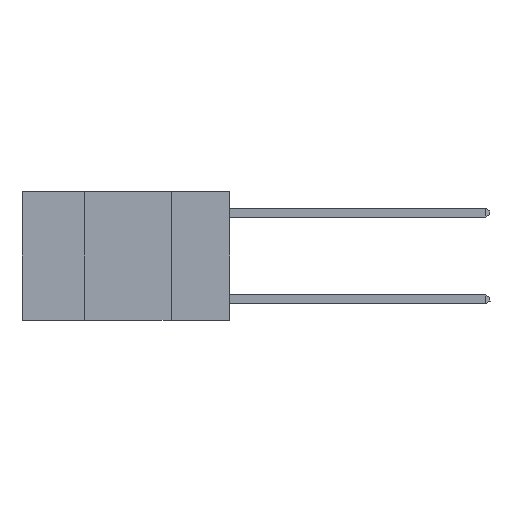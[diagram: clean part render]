
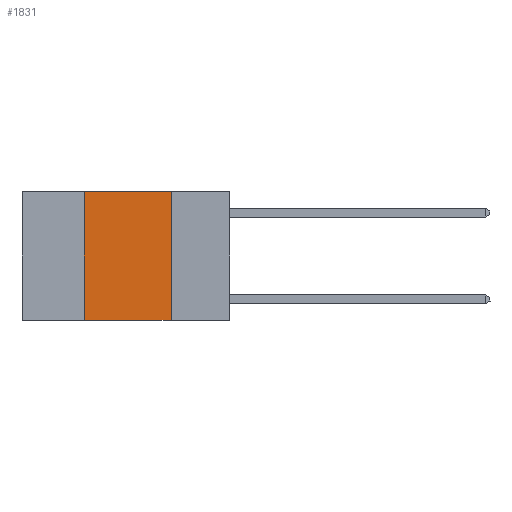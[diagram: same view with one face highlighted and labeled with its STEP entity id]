
A CAD part, left-side view. The second image highlights one B-rep face of the part: STEP entity #1831.
In plain terms, the highlighted planar face has unit normal (-1, 0, 0).
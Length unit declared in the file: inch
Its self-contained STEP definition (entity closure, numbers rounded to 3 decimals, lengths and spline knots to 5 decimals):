
#121 = DIRECTION ( 'NONE',  ( 0., -1., 0. ) ) ;
#196 = ORIENTED_EDGE ( 'NONE', *, *, #12765, .F. ) ;
#263 = ORIENTED_EDGE ( 'NONE', *, *, #1273, .F. ) ;
#486 = EDGE_CURVE ( 'NONE', #14666, #20939, #19412, .T. ) ;
#539 = ORIENTED_EDGE ( 'NONE', *, *, #14400, .F. ) ;
#696 = ORIENTED_EDGE ( 'NONE', *, *, #486, .T. ) ;
#1133 = CARTESIAN_POINT ( 'NONE',  ( 0., 0.42, 0. ) ) ;
#1273 = EDGE_CURVE ( 'NONE', #9100, #5778, #14840, .T. ) ;
#1831 = ADVANCED_FACE ( 'NONE', ( #8430 ), #6531, .F. ) ;
#2457 = CARTESIAN_POINT ( 'NONE',  ( 0., 0.17, 0. ) ) ;
#3127 = CARTESIAN_POINT ( 'NONE',  ( 0., 0.6, 0. ) ) ;
#5778 = VERTEX_POINT ( 'NONE', #11960 ) ;
#6531 = PLANE ( 'NONE',  #10584 ) ;
#8238 = DIRECTION ( 'NONE',  ( 1., 0., 0. ) ) ;
#8430 = FACE_OUTER_BOUND ( 'NONE', #15320, .T. ) ;
#9100 = VERTEX_POINT ( 'NONE', #18956 ) ;
#9338 = LINE ( 'NONE', #2457, #16478 ) ;
#10584 = AXIS2_PLACEMENT_3D ( 'NONE', #3127, #8238, #19606 ) ;
#11960 = CARTESIAN_POINT ( 'NONE',  ( 0., 0.17, 0. ) ) ;
#12765 = EDGE_CURVE ( 'NONE', #5778, #20939, #9338, .T. ) ;
#12866 = DIRECTION ( 'NONE',  ( 0., 0., 1. ) ) ;
#13120 = VECTOR ( 'NONE', #12866, 39.37008 ) ;
#13431 = CARTESIAN_POINT ( 'NONE',  ( 0., 0.42, -0.37 ) ) ;
#14050 = DIRECTION ( 'NONE',  ( 0., -1., 0. ) ) ;
#14340 = VECTOR ( 'NONE', #121, 39.37008 ) ;
#14400 = EDGE_CURVE ( 'NONE', #14666, #9100, #17918, .T. ) ;
#14666 = VERTEX_POINT ( 'NONE', #13431 ) ;
#14840 = LINE ( 'NONE', #17316, #14340 ) ;
#15138 = VECTOR ( 'NONE', #14050, 39.37008 ) ;
#15320 = EDGE_LOOP ( 'NONE', ( #196, #263, #539, #696 ) ) ;
#15321 = CARTESIAN_POINT ( 'NONE',  ( 0., 0.6, -0.37 ) ) ;
#15734 = DIRECTION ( 'NONE',  ( 0., 0., -1. ) ) ;
#16478 = VECTOR ( 'NONE', #15734, 39.37008 ) ;
#17316 = CARTESIAN_POINT ( 'NONE',  ( 0., 0.6, 0. ) ) ;
#17918 = LINE ( 'NONE', #1133, #13120 ) ;
#18956 = CARTESIAN_POINT ( 'NONE',  ( 0., 0.42, 0. ) ) ;
#19412 = LINE ( 'NONE', #15321, #15138 ) ;
#19606 = DIRECTION ( 'NONE',  ( 0., 0., -1. ) ) ;
#19910 = CARTESIAN_POINT ( 'NONE',  ( 0., 0.17, -0.37 ) ) ;
#20939 = VERTEX_POINT ( 'NONE', #19910 ) ;
